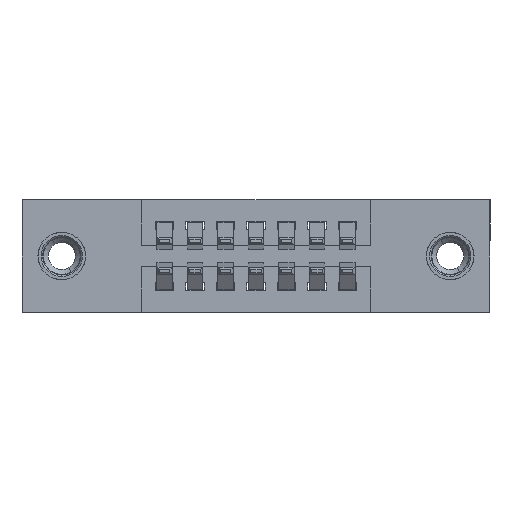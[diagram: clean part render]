
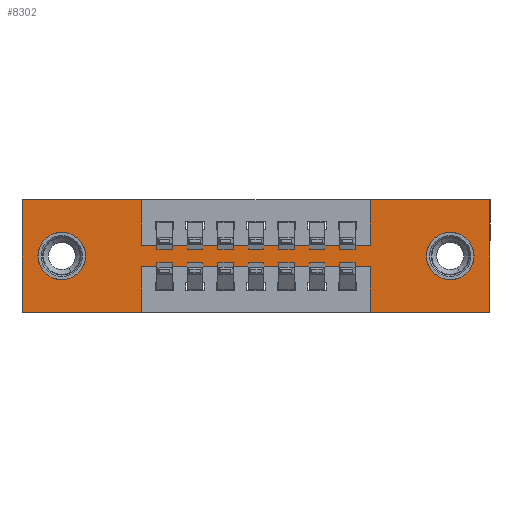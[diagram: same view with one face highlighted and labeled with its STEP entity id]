
A CAD part, front view. The second image highlights one B-rep face of the part: STEP entity #8302.
In plain terms, the highlighted planar face has unit normal (0, -1, 0).
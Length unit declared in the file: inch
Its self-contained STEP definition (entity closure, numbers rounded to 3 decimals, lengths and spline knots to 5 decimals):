
#58 = ORIENTED_EDGE ( 'NONE', *, *, #6758, .F. ) ;
#115 = CARTESIAN_POINT ( 'NONE',  ( 0., 0., -0.37 ) ) ;
#146 = VECTOR ( 'NONE', #2161, 39.37008 ) ;
#187 = VECTOR ( 'NONE', #9330, 39.37008 ) ;
#236 = VERTEX_POINT ( 'NONE', #4175 ) ;
#309 = EDGE_CURVE ( 'NONE', #6178, #6679, #10776, .T. ) ;
#339 = LINE ( 'NONE', #620, #6879 ) ;
#373 = CARTESIAN_POINT ( 'NONE',  ( 0., 0., 0. ) ) ;
#397 = VECTOR ( 'NONE', #1471, 39.37008 ) ;
#488 = CARTESIAN_POINT ( 'NONE',  ( 0.3925, 0., -0.15 ) ) ;
#519 = PLANE ( 'NONE',  #2759 ) ;
#558 = AXIS2_PLACEMENT_3D ( 'NONE', #7954, #6157, #11008 ) ;
#620 = CARTESIAN_POINT ( 'NONE',  ( 0., 0., 0. ) ) ;
#670 = LINE ( 'NONE', #9466, #9700 ) ;
#789 = CARTESIAN_POINT ( 'NONE',  ( 1.1425, 0., 0. ) ) ;
#793 = VECTOR ( 'NONE', #4416, 39.37008 ) ;
#1070 = DIRECTION ( 'NONE',  ( 0., 0., -1. ) ) ;
#1154 = ORIENTED_EDGE ( 'NONE', *, *, #12242, .F. ) ;
#1290 = DIRECTION ( 'NONE',  ( 1., 0., 0. ) ) ;
#1321 = FACE_BOUND ( 'NONE', #1796, .T. ) ;
#1346 = DIRECTION ( 'NONE',  ( 0., 0., -1. ) ) ;
#1471 = DIRECTION ( 'NONE',  ( 0., 0., -1. ) ) ;
#1659 = CIRCLE ( 'NONE', #2246, 0.078 ) ;
#1694 = VERTEX_POINT ( 'NONE', #3722 ) ;
#1702 = ORIENTED_EDGE ( 'NONE', *, *, #309, .F. ) ;
#1796 = EDGE_LOOP ( 'NONE', ( #11522, #2475 ) ) ;
#1984 = VERTEX_POINT ( 'NONE', #4798 ) ;
#2040 = ORIENTED_EDGE ( 'NONE', *, *, #4435, .F. ) ;
#2161 = DIRECTION ( 'NONE',  ( 1., 0., 0. ) ) ;
#2175 = EDGE_CURVE ( 'NONE', #5717, #5409, #4302, .T. ) ;
#2246 = AXIS2_PLACEMENT_3D ( 'NONE', #3458, #6277, #8294 ) ;
#2317 = VECTOR ( 'NONE', #4306, 39.37008 ) ;
#2398 = LINE ( 'NONE', #3010, #12384 ) ;
#2475 = ORIENTED_EDGE ( 'NONE', *, *, #12360, .T. ) ;
#2514 = VERTEX_POINT ( 'NONE', #5130 ) ;
#2627 = VERTEX_POINT ( 'NONE', #4601 ) ;
#2759 = AXIS2_PLACEMENT_3D ( 'NONE', #5224, #11053, #6243 ) ;
#2873 = EDGE_CURVE ( 'NONE', #6584, #236, #8085, .T. ) ;
#2938 = DIRECTION ( 'NONE',  ( 0., 0., -1. ) ) ;
#3010 = CARTESIAN_POINT ( 'NONE',  ( 1.535, 0., 0. ) ) ;
#3147 = CARTESIAN_POINT ( 'NONE',  ( 0.13, 0., -0.185 ) ) ;
#3195 = DIRECTION ( 'NONE',  ( 0., 1., 0. ) ) ;
#3330 = ORIENTED_EDGE ( 'NONE', *, *, #2873, .F. ) ;
#3458 = CARTESIAN_POINT ( 'NONE',  ( 1.405, 0., -0.185 ) ) ;
#3504 = CARTESIAN_POINT ( 'NONE',  ( 0.3925, 0., -0.22 ) ) ;
#3722 = CARTESIAN_POINT ( 'NONE',  ( 0.3925, 0., -0.37 ) ) ;
#3839 = DIRECTION ( 'NONE',  ( 0., 1., 0. ) ) ;
#4175 = CARTESIAN_POINT ( 'NONE',  ( 1.1425, 0., -0.15 ) ) ;
#4240 = EDGE_CURVE ( 'NONE', #8128, #10446, #6366, .T. ) ;
#4294 = CARTESIAN_POINT ( 'NONE',  ( 0., 0., -0.37 ) ) ;
#4302 = LINE ( 'NONE', #6868, #146 ) ;
#4306 = DIRECTION ( 'NONE',  ( 0., 0., 1. ) ) ;
#4416 = DIRECTION ( 'NONE',  ( -1., 0., 0. ) ) ;
#4428 = EDGE_LOOP ( 'NONE', ( #12073, #1154, #1702, #5318, #58, #11115, #8312, #3330, #2040, #4454, #6263, #9739 ) ) ;
#4435 = EDGE_CURVE ( 'NONE', #5409, #6584, #670, .T. ) ;
#4454 = ORIENTED_EDGE ( 'NONE', *, *, #2175, .F. ) ;
#4601 = CARTESIAN_POINT ( 'NONE',  ( 1.405, 0., -0.107 ) ) ;
#4753 = CARTESIAN_POINT ( 'NONE',  ( 1.1425, 0., 0. ) ) ;
#4798 = CARTESIAN_POINT ( 'NONE',  ( 0., 0., -0.37 ) ) ;
#4834 = CARTESIAN_POINT ( 'NONE',  ( 1.535, 0., 0. ) ) ;
#4941 = VERTEX_POINT ( 'NONE', #5507 ) ;
#5107 = EDGE_LOOP ( 'NONE', ( #7681, #9308 ) ) ;
#5130 = CARTESIAN_POINT ( 'NONE',  ( 1.535, 0., -0.37 ) ) ;
#5224 = CARTESIAN_POINT ( 'NONE',  ( 0., 0., -0.37 ) ) ;
#5318 = ORIENTED_EDGE ( 'NONE', *, *, #10437, .F. ) ;
#5409 = VERTEX_POINT ( 'NONE', #10192 ) ;
#5507 = CARTESIAN_POINT ( 'NONE',  ( 0.13, 0., -0.263 ) ) ;
#5684 = AXIS2_PLACEMENT_3D ( 'NONE', #3147, #3195, #9967 ) ;
#5717 = VERTEX_POINT ( 'NONE', #373 ) ;
#5886 = LINE ( 'NONE', #4294, #793 ) ;
#6095 = CARTESIAN_POINT ( 'NONE',  ( 0., 0., 0. ) ) ;
#6157 = DIRECTION ( 'NONE',  ( 0., 1., 0. ) ) ;
#6178 = VERTEX_POINT ( 'NONE', #10542 ) ;
#6243 = DIRECTION ( 'NONE',  ( 0., 0., -1. ) ) ;
#6263 = ORIENTED_EDGE ( 'NONE', *, *, #8566, .F. ) ;
#6277 = DIRECTION ( 'NONE',  ( 0., 1., 0. ) ) ;
#6366 = LINE ( 'NONE', #6095, #10925 ) ;
#6425 = EDGE_CURVE ( 'NONE', #236, #8128, #10713, .T. ) ;
#6584 = VERTEX_POINT ( 'NONE', #8970 ) ;
#6591 = LINE ( 'NONE', #6965, #9947 ) ;
#6679 = VERTEX_POINT ( 'NONE', #11742 ) ;
#6758 = EDGE_CURVE ( 'NONE', #10446, #2514, #2398, .T. ) ;
#6868 = CARTESIAN_POINT ( 'NONE',  ( 0., 0., 0. ) ) ;
#6879 = VECTOR ( 'NONE', #8412, 39.37008 ) ;
#6965 = CARTESIAN_POINT ( 'NONE',  ( 0.3925, 0., -0.22 ) ) ;
#7170 = VERTEX_POINT ( 'NONE', #3504 ) ;
#7379 = CARTESIAN_POINT ( 'NONE',  ( 1.1425, 0., -0.37 ) ) ;
#7509 = FACE_BOUND ( 'NONE', #5107, .T. ) ;
#7636 = AXIS2_PLACEMENT_3D ( 'NONE', #11613, #3839, #1070 ) ;
#7681 = ORIENTED_EDGE ( 'NONE', *, *, #9237, .T. ) ;
#7954 = CARTESIAN_POINT ( 'NONE',  ( 0.13, 0., -0.185 ) ) ;
#7990 = VERTEX_POINT ( 'NONE', #12273 ) ;
#8085 = LINE ( 'NONE', #488, #8260 ) ;
#8128 = VERTEX_POINT ( 'NONE', #4753 ) ;
#8204 = CIRCLE ( 'NONE', #558, 0.078 ) ;
#8260 = VECTOR ( 'NONE', #1290, 39.37008 ) ;
#8294 = DIRECTION ( 'NONE',  ( 0., 0., -1. ) ) ;
#8302 = ADVANCED_FACE ( 'NONE', ( #1321, #7509, #10397 ), #519, .T. ) ;
#8312 = ORIENTED_EDGE ( 'NONE', *, *, #6425, .F. ) ;
#8412 = DIRECTION ( 'NONE',  ( 0., 0., 1. ) ) ;
#8566 = EDGE_CURVE ( 'NONE', #1984, #5717, #339, .T. ) ;
#8634 = VECTOR ( 'NONE', #8868, 39.37008 ) ;
#8769 = LINE ( 'NONE', #115, #8634 ) ;
#8795 = EDGE_CURVE ( 'NONE', #7170, #1694, #10616, .T. ) ;
#8868 = DIRECTION ( 'NONE',  ( -1., 0., 0. ) ) ;
#8970 = CARTESIAN_POINT ( 'NONE',  ( 0.3925, 0., -0.15 ) ) ;
#9237 = EDGE_CURVE ( 'NONE', #12019, #4941, #8204, .T. ) ;
#9308 = ORIENTED_EDGE ( 'NONE', *, *, #10036, .T. ) ;
#9330 = DIRECTION ( 'NONE',  ( 0., 0., 1. ) ) ;
#9466 = CARTESIAN_POINT ( 'NONE',  ( 0.3925, 0., 0. ) ) ;
#9491 = CARTESIAN_POINT ( 'NONE',  ( 0.13, 0., -0.107 ) ) ;
#9700 = VECTOR ( 'NONE', #2938, 39.37008 ) ;
#9739 = ORIENTED_EDGE ( 'NONE', *, *, #10653, .F. ) ;
#9947 = VECTOR ( 'NONE', #10822, 39.37008 ) ;
#9967 = DIRECTION ( 'NONE',  ( 0., 0., 1. ) ) ;
#10036 = EDGE_CURVE ( 'NONE', #4941, #12019, #10335, .T. ) ;
#10192 = CARTESIAN_POINT ( 'NONE',  ( 0.3925, 0., 0. ) ) ;
#10335 = CIRCLE ( 'NONE', #5684, 0.078 ) ;
#10397 = FACE_OUTER_BOUND ( 'NONE', #4428, .T. ) ;
#10398 = EDGE_CURVE ( 'NONE', #2627, #7990, #11377, .T. ) ;
#10437 = EDGE_CURVE ( 'NONE', #2514, #6178, #8769, .T. ) ;
#10446 = VERTEX_POINT ( 'NONE', #4834 ) ;
#10542 = CARTESIAN_POINT ( 'NONE',  ( 1.1425, 0., -0.37 ) ) ;
#10616 = LINE ( 'NONE', #10917, #397 ) ;
#10653 = EDGE_CURVE ( 'NONE', #1694, #1984, #5886, .T. ) ;
#10713 = LINE ( 'NONE', #789, #187 ) ;
#10776 = LINE ( 'NONE', #7379, #2317 ) ;
#10822 = DIRECTION ( 'NONE',  ( -1., 0., 0. ) ) ;
#10917 = CARTESIAN_POINT ( 'NONE',  ( 0.3925, 0., -0.37 ) ) ;
#10925 = VECTOR ( 'NONE', #11965, 39.37008 ) ;
#11008 = DIRECTION ( 'NONE',  ( 0., 0., 1. ) ) ;
#11053 = DIRECTION ( 'NONE',  ( 0., -1., 0. ) ) ;
#11115 = ORIENTED_EDGE ( 'NONE', *, *, #4240, .F. ) ;
#11377 = CIRCLE ( 'NONE', #7636, 0.078 ) ;
#11522 = ORIENTED_EDGE ( 'NONE', *, *, #10398, .T. ) ;
#11613 = CARTESIAN_POINT ( 'NONE',  ( 1.405, 0., -0.185 ) ) ;
#11742 = CARTESIAN_POINT ( 'NONE',  ( 1.1425, 0., -0.22 ) ) ;
#11965 = DIRECTION ( 'NONE',  ( 1., 0., 0. ) ) ;
#12019 = VERTEX_POINT ( 'NONE', #9491 ) ;
#12073 = ORIENTED_EDGE ( 'NONE', *, *, #8795, .F. ) ;
#12242 = EDGE_CURVE ( 'NONE', #6679, #7170, #6591, .T. ) ;
#12273 = CARTESIAN_POINT ( 'NONE',  ( 1.405, 0., -0.263 ) ) ;
#12360 = EDGE_CURVE ( 'NONE', #7990, #2627, #1659, .T. ) ;
#12384 = VECTOR ( 'NONE', #1346, 39.37008 ) ;
